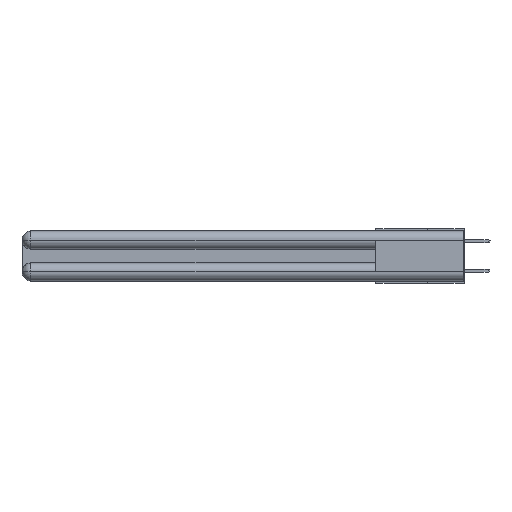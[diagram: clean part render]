
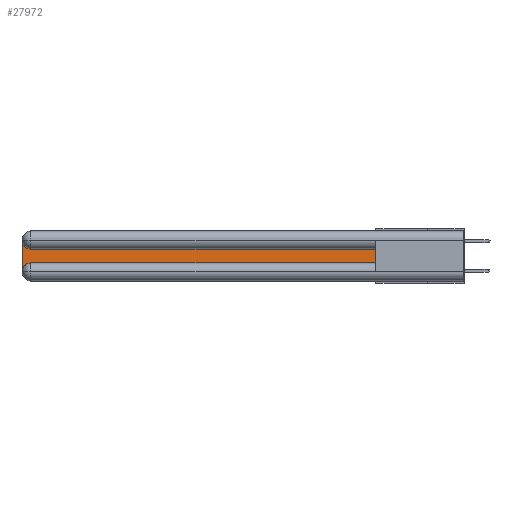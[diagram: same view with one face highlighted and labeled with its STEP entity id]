
A CAD part, left-side view. The second image highlights one B-rep face of the part: STEP entity #27972.
In plain terms, the highlighted planar face has unit normal (-1, 0, 0).
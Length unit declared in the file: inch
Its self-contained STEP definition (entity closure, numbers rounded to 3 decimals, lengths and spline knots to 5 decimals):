
#217 = CARTESIAN_POINT ( 'NONE',  ( 0.075, 2.94, -0.2775 ) ) ;
#2699 = VERTEX_POINT ( 'NONE', #12743 ) ;
#3677 = DIRECTION ( 'NONE',  ( 0., 0., -1. ) ) ;
#3762 = CARTESIAN_POINT ( 'NONE',  ( 0.075, 3., -0.2175 ) ) ;
#3864 = PLANE ( 'NONE',  #25870 ) ;
#3961 = EDGE_LOOP ( 'NONE', ( #10608, #22381, #22656, #9194, #14721, #12377 ) ) ;
#3966 = DIRECTION ( 'NONE',  ( 1., 0., 0. ) ) ;
#4171 = CARTESIAN_POINT ( 'NONE',  ( 0.075, 3., -0.2775 ) ) ;
#5258 = LINE ( 'NONE', #9833, #6279 ) ;
#5909 = VECTOR ( 'NONE', #24115, 39.37008 ) ;
#5958 = DIRECTION ( 'NONE',  ( 0., 0., -1. ) ) ;
#6061 = CARTESIAN_POINT ( 'NONE',  ( 0.075, 2.94, -0.0625 ) ) ;
#6279 = VECTOR ( 'NONE', #27247, 39.37008 ) ;
#6775 = CARTESIAN_POINT ( 'NONE',  ( 0.075, 0.6, -0.1225 ) ) ;
#7055 = VECTOR ( 'NONE', #22036, 39.37008 ) ;
#7202 = CARTESIAN_POINT ( 'NONE',  ( 0.075, 3., -0.0625 ) ) ;
#7545 = EDGE_CURVE ( 'NONE', #14430, #2699, #14758, .T. ) ;
#9147 = DIRECTION ( 'NONE',  ( 0., 0., -1. ) ) ;
#9194 = ORIENTED_EDGE ( 'NONE', *, *, #7545, .T. ) ;
#9370 = CARTESIAN_POINT ( 'NONE',  ( 0.075, 0.6, -0.2175 ) ) ;
#9459 = EDGE_CURVE ( 'NONE', #20062, #14430, #13127, .T. ) ;
#9680 = LINE ( 'NONE', #20113, #5909 ) ;
#9833 = CARTESIAN_POINT ( 'NONE',  ( 0.075, 0.6, -0.2175 ) ) ;
#9860 = EDGE_CURVE ( 'NONE', #18845, #23652, #5258, .T. ) ;
#10608 = ORIENTED_EDGE ( 'NONE', *, *, #14801, .T. ) ;
#11215 = CARTESIAN_POINT ( 'NONE',  ( 0.075, 2.94, -0.1225 ) ) ;
#11248 = DIRECTION ( 'NONE',  ( 1., 0., 0. ) ) ;
#11765 = EDGE_CURVE ( 'NONE', #22166, #20062, #15750, .T. ) ;
#12377 = ORIENTED_EDGE ( 'NONE', *, *, #9860, .T. ) ;
#12548 = DIRECTION ( 'NONE',  ( 1., 0., 0. ) ) ;
#12637 = DIRECTION ( 'NONE',  ( 0., 0., -1. ) ) ;
#12743 = CARTESIAN_POINT ( 'NONE',  ( 0.075, 2.94, -0.2175 ) ) ;
#13127 = LINE ( 'NONE', #3762, #25034 ) ;
#13667 = AXIS2_PLACEMENT_3D ( 'NONE', #217, #11248, #9147 ) ;
#14430 = VERTEX_POINT ( 'NONE', #4171 ) ;
#14721 = ORIENTED_EDGE ( 'NONE', *, *, #19352, .T. ) ;
#14758 = CIRCLE ( 'NONE', #13667, 0.06 ) ;
#14801 = EDGE_CURVE ( 'NONE', #23652, #22166, #25805, .T. ) ;
#15750 = CIRCLE ( 'NONE', #16685, 0.06 ) ;
#16685 = AXIS2_PLACEMENT_3D ( 'NONE', #6061, #3966, #12637 ) ;
#18462 = CARTESIAN_POINT ( 'NONE',  ( 0.075, 0.6, -0.1225 ) ) ;
#18845 = VERTEX_POINT ( 'NONE', #9370 ) ;
#19352 = EDGE_CURVE ( 'NONE', #2699, #18845, #9680, .T. ) ;
#20062 = VERTEX_POINT ( 'NONE', #7202 ) ;
#20113 = CARTESIAN_POINT ( 'NONE',  ( 0.075, 0.6, -0.2175 ) ) ;
#22036 = DIRECTION ( 'NONE',  ( 0., 1., 0. ) ) ;
#22166 = VERTEX_POINT ( 'NONE', #11215 ) ;
#22381 = ORIENTED_EDGE ( 'NONE', *, *, #11765, .T. ) ;
#22656 = ORIENTED_EDGE ( 'NONE', *, *, #9459, .T. ) ;
#23652 = VERTEX_POINT ( 'NONE', #18462 ) ;
#24115 = DIRECTION ( 'NONE',  ( 0., -1., 0. ) ) ;
#25034 = VECTOR ( 'NONE', #5958, 39.37008 ) ;
#25589 = CARTESIAN_POINT ( 'NONE',  ( 0.075, 3., -0.1225 ) ) ;
#25805 = LINE ( 'NONE', #6775, #7055 ) ;
#25870 = AXIS2_PLACEMENT_3D ( 'NONE', #25589, #12548, #3677 ) ;
#27247 = DIRECTION ( 'NONE',  ( 0., 0., 1. ) ) ;
#27654 = FACE_OUTER_BOUND ( 'NONE', #3961, .T. ) ;
#27972 = ADVANCED_FACE ( 'NONE', ( #27654 ), #3864, .F. ) ;
